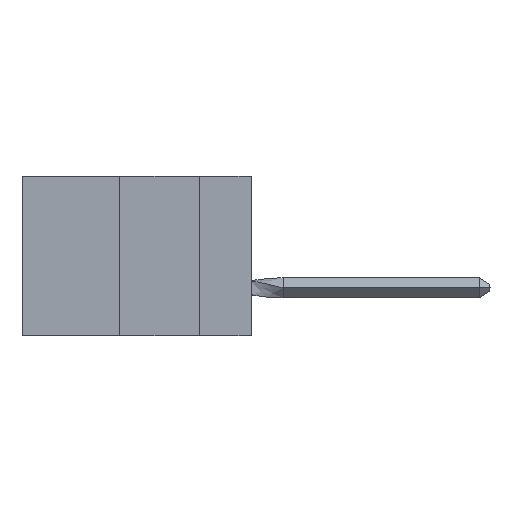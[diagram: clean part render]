
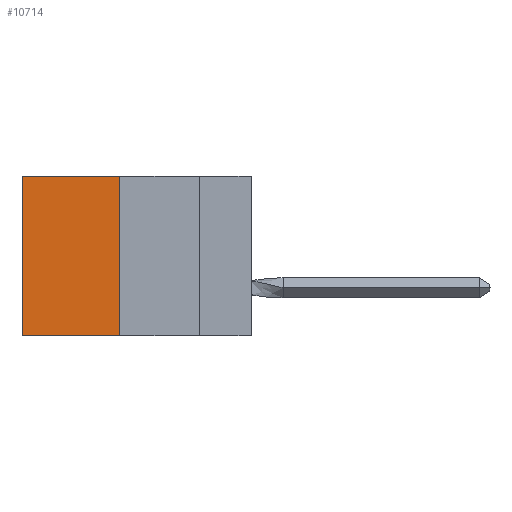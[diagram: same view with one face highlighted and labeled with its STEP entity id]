
A CAD part, left-side view. The second image highlights one B-rep face of the part: STEP entity #10714.
In plain terms, the highlighted planar face has unit normal (-1, 0, 0).
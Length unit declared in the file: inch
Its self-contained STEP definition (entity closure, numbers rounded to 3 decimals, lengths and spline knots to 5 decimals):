
#34 = ORIENTED_EDGE ( 'NONE', *, *, #9742, .T. ) ;
#129 = DIRECTION ( 'NONE',  ( 0., 0., -1. ) ) ;
#800 = VERTEX_POINT ( 'NONE', #1229 ) ;
#1229 = CARTESIAN_POINT ( 'NONE',  ( 0.305, 0.413, -0.5 ) ) ;
#1366 = EDGE_CURVE ( 'NONE', #9468, #6696, #10327, .T. ) ;
#1371 = EDGE_LOOP ( 'NONE', ( #34, #2898, #1960, #8700 ) ) ;
#1529 = CARTESIAN_POINT ( 'NONE',  ( 0.305, 0.413, 0. ) ) ;
#1737 = PLANE ( 'NONE',  #4364 ) ;
#1913 = VECTOR ( 'NONE', #11143, 39.37008 ) ;
#1960 = ORIENTED_EDGE ( 'NONE', *, *, #11588, .F. ) ;
#2856 = LINE ( 'NONE', #3875, #8916 ) ;
#2898 = ORIENTED_EDGE ( 'NONE', *, *, #2994, .F. ) ;
#2994 = EDGE_CURVE ( 'NONE', #800, #4150, #2856, .T. ) ;
#3190 = CARTESIAN_POINT ( 'NONE',  ( 0.305, 0.413, -0.5 ) ) ;
#3402 = CARTESIAN_POINT ( 'NONE',  ( 0.305, 0.72, -0.5 ) ) ;
#3875 = CARTESIAN_POINT ( 'NONE',  ( 0.305, 0.413, -0.5 ) ) ;
#4150 = VERTEX_POINT ( 'NONE', #3402 ) ;
#4364 = AXIS2_PLACEMENT_3D ( 'NONE', #6563, #8383, #12265 ) ;
#4979 = DIRECTION ( 'NONE',  ( 0., 1., 0. ) ) ;
#5321 = VECTOR ( 'NONE', #10250, 39.37008 ) ;
#5403 = LINE ( 'NONE', #10224, #1913 ) ;
#6563 = CARTESIAN_POINT ( 'NONE',  ( 0.305, 0.413, -0.5 ) ) ;
#6696 = VERTEX_POINT ( 'NONE', #6987 ) ;
#6987 = CARTESIAN_POINT ( 'NONE',  ( 0.305, 0.72, 0. ) ) ;
#7770 = LINE ( 'NONE', #3190, #12438 ) ;
#7794 = FACE_OUTER_BOUND ( 'NONE', #1371, .T. ) ;
#8383 = DIRECTION ( 'NONE',  ( 1., 0., 0. ) ) ;
#8700 = ORIENTED_EDGE ( 'NONE', *, *, #1366, .T. ) ;
#8916 = VECTOR ( 'NONE', #4979, 39.37008 ) ;
#9468 = VERTEX_POINT ( 'NONE', #11344 ) ;
#9742 = EDGE_CURVE ( 'NONE', #6696, #4150, #5403, .T. ) ;
#10224 = CARTESIAN_POINT ( 'NONE',  ( 0.305, 0.72, -0.5 ) ) ;
#10250 = DIRECTION ( 'NONE',  ( 0., 1., 0. ) ) ;
#10327 = LINE ( 'NONE', #1529, #5321 ) ;
#10714 = ADVANCED_FACE ( 'NONE', ( #7794 ), #1737, .F. ) ;
#11143 = DIRECTION ( 'NONE',  ( 0., 0., -1. ) ) ;
#11344 = CARTESIAN_POINT ( 'NONE',  ( 0.305, 0.413, 0. ) ) ;
#11588 = EDGE_CURVE ( 'NONE', #9468, #800, #7770, .T. ) ;
#12265 = DIRECTION ( 'NONE',  ( 0., 0., -1. ) ) ;
#12438 = VECTOR ( 'NONE', #129, 39.37008 ) ;
